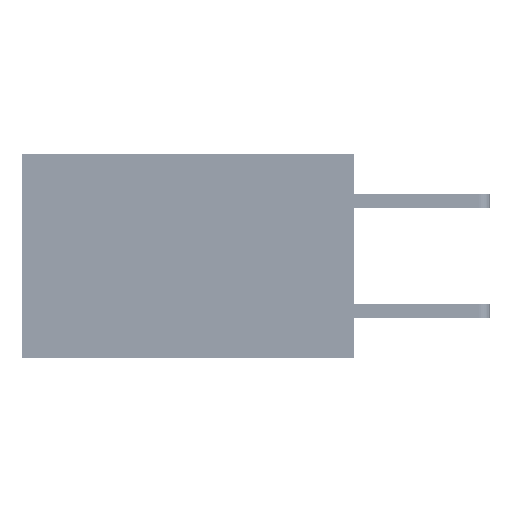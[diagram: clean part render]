
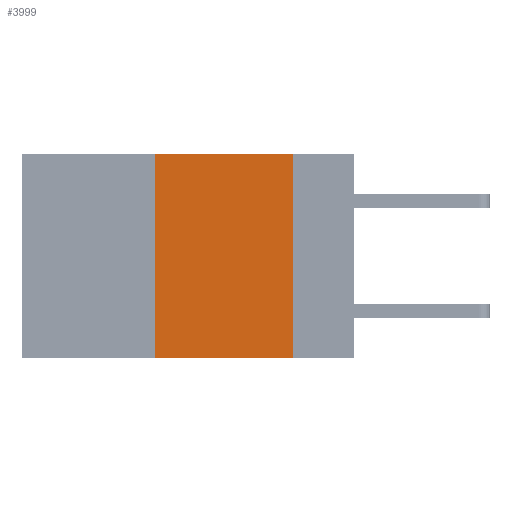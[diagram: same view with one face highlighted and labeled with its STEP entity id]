
A CAD part, left-side view. The second image highlights one B-rep face of the part: STEP entity #3999.
In plain terms, the highlighted planar face has unit normal (-1, 0, 0).
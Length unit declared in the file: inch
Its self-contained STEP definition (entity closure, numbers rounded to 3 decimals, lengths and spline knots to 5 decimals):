
#182 = ORIENTED_EDGE ( 'NONE', *, *, #5324, .F. ) ;
#3999 = ADVANCED_FACE ( 'NONE', ( #13089 ), #32003, .F. ) ;
#4132 = ORIENTED_EDGE ( 'NONE', *, *, #49556, .F. ) ;
#5324 = EDGE_CURVE ( 'NONE', #43922, #20999, #19833, .T. ) ;
#6297 = VECTOR ( 'NONE', #12202, 39.37008 ) ;
#6430 = DIRECTION ( 'NONE',  ( 0., 0., 1. ) ) ;
#8838 = DIRECTION ( 'NONE',  ( 0., -1., 0. ) ) ;
#12202 = DIRECTION ( 'NONE',  ( 0., 0., -1. ) ) ;
#13089 = FACE_OUTER_BOUND ( 'NONE', #41717, .T. ) ;
#14434 = CARTESIAN_POINT ( 'NONE',  ( 0., 0.6, -0.37 ) ) ;
#14498 = CARTESIAN_POINT ( 'NONE',  ( 0., 0.11, -0.37 ) ) ;
#14891 = EDGE_CURVE ( 'NONE', #49917, #18856, #31802, .T. ) ;
#16598 = DIRECTION ( 'NONE',  ( 0., 0., -1. ) ) ;
#16938 = LINE ( 'NONE', #48092, #6297 ) ;
#16973 = ORIENTED_EDGE ( 'NONE', *, *, #14891, .T. ) ;
#18856 = VERTEX_POINT ( 'NONE', #14498 ) ;
#19833 = LINE ( 'NONE', #48737, #36086 ) ;
#20629 = CARTESIAN_POINT ( 'NONE',  ( 0., 0.6, 0. ) ) ;
#20999 = VERTEX_POINT ( 'NONE', #23632 ) ;
#21414 = VECTOR ( 'NONE', #6430, 39.37008 ) ;
#21629 = EDGE_CURVE ( 'NONE', #20999, #18856, #16938, .T. ) ;
#22483 = DIRECTION ( 'NONE',  ( 0., -1., 0. ) ) ;
#23632 = CARTESIAN_POINT ( 'NONE',  ( 0., 0.11, 0. ) ) ;
#31802 = LINE ( 'NONE', #14434, #33048 ) ;
#32003 = PLANE ( 'NONE',  #36122 ) ;
#33048 = VECTOR ( 'NONE', #22483, 39.37008 ) ;
#34402 = CARTESIAN_POINT ( 'NONE',  ( 0., 0.36, 0. ) ) ;
#36086 = VECTOR ( 'NONE', #8838, 39.37008 ) ;
#36122 = AXIS2_PLACEMENT_3D ( 'NONE', #20629, #48454, #16598 ) ;
#38131 = ORIENTED_EDGE ( 'NONE', *, *, #21629, .F. ) ;
#41180 = CARTESIAN_POINT ( 'NONE',  ( 0., 0.36, -0.37 ) ) ;
#41717 = EDGE_LOOP ( 'NONE', ( #38131, #182, #4132, #16973 ) ) ;
#42714 = LINE ( 'NONE', #34402, #21414 ) ;
#43922 = VERTEX_POINT ( 'NONE', #46819 ) ;
#46819 = CARTESIAN_POINT ( 'NONE',  ( 0., 0.36, 0. ) ) ;
#48092 = CARTESIAN_POINT ( 'NONE',  ( 0., 0.11, 0. ) ) ;
#48454 = DIRECTION ( 'NONE',  ( 1., 0., 0. ) ) ;
#48737 = CARTESIAN_POINT ( 'NONE',  ( 0., 0.6, 0. ) ) ;
#49556 = EDGE_CURVE ( 'NONE', #49917, #43922, #42714, .T. ) ;
#49917 = VERTEX_POINT ( 'NONE', #41180 ) ;
